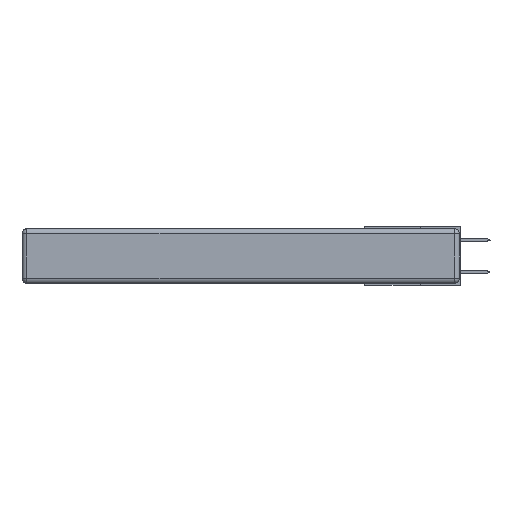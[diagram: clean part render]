
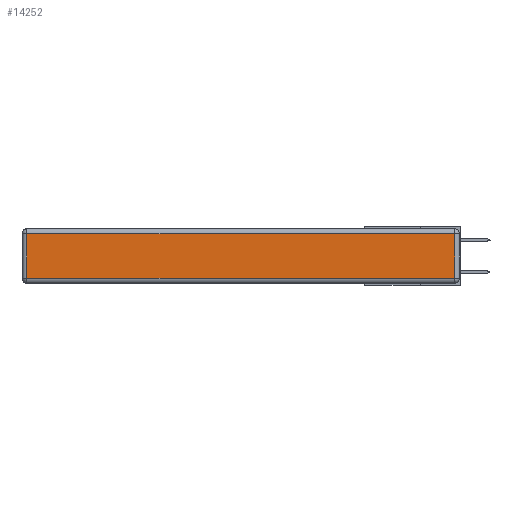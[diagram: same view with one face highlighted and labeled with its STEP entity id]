
A CAD part, left-side view. The second image highlights one B-rep face of the part: STEP entity #14252.
In plain terms, the highlighted planar face has unit normal (-1, 0, 0).
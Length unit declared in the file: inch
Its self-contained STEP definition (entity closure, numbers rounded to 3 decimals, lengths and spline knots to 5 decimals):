
#16 = VECTOR ( 'NONE', #18592, 39.37008 ) ;
#64 = LINE ( 'NONE', #18017, #5736 ) ;
#1386 = CARTESIAN_POINT ( 'NONE',  ( 0., 2.72, -0.343 ) ) ;
#1972 = LINE ( 'NONE', #12045, #20578 ) ;
#3838 = VERTEX_POINT ( 'NONE', #10667 ) ;
#3900 = VECTOR ( 'NONE', #7610, 39.37008 ) ;
#5122 = CARTESIAN_POINT ( 'NONE',  ( 0., 0.03, -0.313 ) ) ;
#5736 = VECTOR ( 'NONE', #20136, 39.37008 ) ;
#5923 = EDGE_CURVE ( 'NONE', #15335, #3838, #6579, .T. ) ;
#5939 = EDGE_CURVE ( 'NONE', #3838, #18622, #19536, .T. ) ;
#6579 = LINE ( 'NONE', #14622, #16 ) ;
#7610 = DIRECTION ( 'NONE',  ( 0., 0., -1. ) ) ;
#7915 = CARTESIAN_POINT ( 'NONE',  ( 0., 0.03, -0.03 ) ) ;
#8104 = EDGE_CURVE ( 'NONE', #8825, #15335, #1972, .T. ) ;
#8825 = VERTEX_POINT ( 'NONE', #5122 ) ;
#9389 = FACE_OUTER_BOUND ( 'NONE', #17722, .T. ) ;
#10487 = DIRECTION ( 'NONE',  ( 0., 0., 1. ) ) ;
#10667 = CARTESIAN_POINT ( 'NONE',  ( 0., 2.72, -0.03 ) ) ;
#11483 = AXIS2_PLACEMENT_3D ( 'NONE', #18085, #22019, #10487 ) ;
#12045 = CARTESIAN_POINT ( 'NONE',  ( 0., 0.03, -0.343 ) ) ;
#14000 = DIRECTION ( 'NONE',  ( 0., 0., 1. ) ) ;
#14252 = ADVANCED_FACE ( 'NONE', ( #9389 ), #14530, .T. ) ;
#14530 = PLANE ( 'NONE',  #11483 ) ;
#14622 = CARTESIAN_POINT ( 'NONE',  ( 0., 2.75, -0.03 ) ) ;
#15335 = VERTEX_POINT ( 'NONE', #7915 ) ;
#15957 = ORIENTED_EDGE ( 'NONE', *, *, #5923, .T. ) ;
#17722 = EDGE_LOOP ( 'NONE', ( #23523, #18070, #15957, #20063 ) ) ;
#18017 = CARTESIAN_POINT ( 'NONE',  ( 0., 0., -0.313 ) ) ;
#18070 = ORIENTED_EDGE ( 'NONE', *, *, #8104, .T. ) ;
#18085 = CARTESIAN_POINT ( 'NONE',  ( 0., 0., -0.343 ) ) ;
#18592 = DIRECTION ( 'NONE',  ( 0., 1., 0. ) ) ;
#18622 = VERTEX_POINT ( 'NONE', #22945 ) ;
#19536 = LINE ( 'NONE', #1386, #3900 ) ;
#20063 = ORIENTED_EDGE ( 'NONE', *, *, #5939, .T. ) ;
#20136 = DIRECTION ( 'NONE',  ( 0., -1., 0. ) ) ;
#20578 = VECTOR ( 'NONE', #14000, 39.37008 ) ;
#22019 = DIRECTION ( 'NONE',  ( -1., 0., 0. ) ) ;
#22945 = CARTESIAN_POINT ( 'NONE',  ( 0., 2.72, -0.313 ) ) ;
#23131 = EDGE_CURVE ( 'NONE', #18622, #8825, #64, .T. ) ;
#23523 = ORIENTED_EDGE ( 'NONE', *, *, #23131, .T. ) ;
